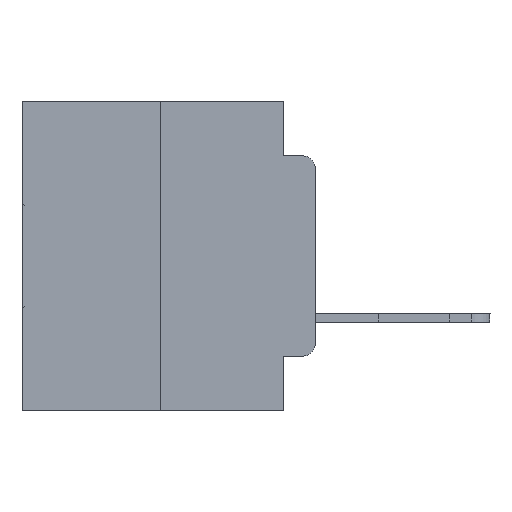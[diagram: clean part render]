
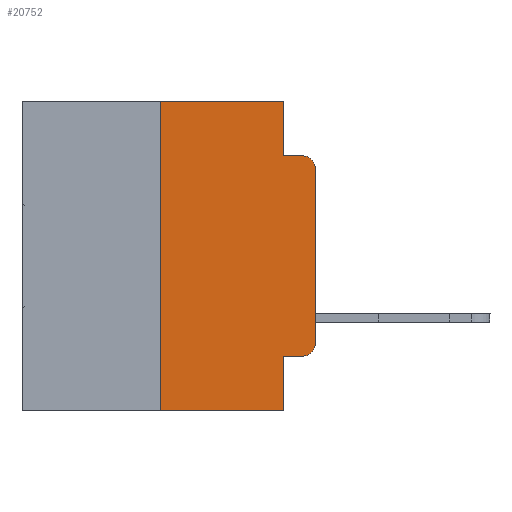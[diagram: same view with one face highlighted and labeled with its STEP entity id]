
A CAD part, left-side view. The second image highlights one B-rep face of the part: STEP entity #20752.
In plain terms, the highlighted planar face has unit normal (-1, 0, 0).
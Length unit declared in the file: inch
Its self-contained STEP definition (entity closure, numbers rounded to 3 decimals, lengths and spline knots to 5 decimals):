
#419 = CARTESIAN_POINT ( 'NONE',  ( 0., 0.25, 0. ) ) ;
#606 = CARTESIAN_POINT ( 'NONE',  ( 0., 0., -0.3915 ) ) ;
#669 = CARTESIAN_POINT ( 'NONE',  ( 0., 0.051, 0. ) ) ;
#804 = LINE ( 'NONE', #19775, #17486 ) ;
#951 = DIRECTION ( 'NONE',  ( 0., 0., 1. ) ) ;
#1592 = CIRCLE ( 'NONE', #18840, 0.02 ) ;
#1595 = VERTEX_POINT ( 'NONE', #11694 ) ;
#1695 = AXIS2_PLACEMENT_3D ( 'NONE', #17383, #21545, #22154 ) ;
#1738 = DIRECTION ( 'NONE',  ( 0., -1., 0. ) ) ;
#2549 = VERTEX_POINT ( 'NONE', #7487 ) ;
#3279 = DIRECTION ( 'NONE',  ( 0., -1., 0. ) ) ;
#3861 = LINE ( 'NONE', #10783, #11491 ) ;
#3958 = DIRECTION ( 'NONE',  ( 0., 0., -1. ) ) ;
#3966 = AXIS2_PLACEMENT_3D ( 'NONE', #23232, #30220, #18471 ) ;
#4271 = EDGE_CURVE ( 'NONE', #17627, #30252, #14531, .T. ) ;
#4440 = VECTOR ( 'NONE', #3279, 39.37008 ) ;
#4605 = EDGE_LOOP ( 'NONE', ( #21829, #26797, #7117, #13306, #5757, #14595, #7128, #30144, #10093, #21028 ) ) ;
#4985 = EDGE_CURVE ( 'NONE', #2549, #11562, #25563, .T. ) ;
#5744 = LINE ( 'NONE', #22222, #4440 ) ;
#5757 = ORIENTED_EDGE ( 'NONE', *, *, #18303, .F. ) ;
#5864 = VECTOR ( 'NONE', #15097, 39.37008 ) ;
#5902 = EDGE_CURVE ( 'NONE', #30252, #1595, #30450, .T. ) ;
#6828 = DIRECTION ( 'NONE',  ( 0., -1., 0. ) ) ;
#7117 = ORIENTED_EDGE ( 'NONE', *, *, #5902, .F. ) ;
#7128 = ORIENTED_EDGE ( 'NONE', *, *, #15483, .T. ) ;
#7487 = CARTESIAN_POINT ( 'NONE',  ( 0., 0.02, -0.4115 ) ) ;
#7666 = FACE_OUTER_BOUND ( 'NONE', #4605, .T. ) ;
#8427 = CARTESIAN_POINT ( 'NONE',  ( 0., 0.02, -0.1085 ) ) ;
#9106 = EDGE_CURVE ( 'NONE', #24714, #1595, #1592, .T. ) ;
#10093 = ORIENTED_EDGE ( 'NONE', *, *, #13105, .T. ) ;
#10783 = CARTESIAN_POINT ( 'NONE',  ( 0., 0.25, 0. ) ) ;
#10971 = CARTESIAN_POINT ( 'NONE',  ( 0., 0.473, -0.5 ) ) ;
#11491 = VECTOR ( 'NONE', #22671, 39.37008 ) ;
#11562 = VERTEX_POINT ( 'NONE', #606 ) ;
#11694 = CARTESIAN_POINT ( 'NONE',  ( 0., 0.02, -0.0885 ) ) ;
#11901 = DIRECTION ( 'NONE',  ( 0., 0., -1. ) ) ;
#13105 = EDGE_CURVE ( 'NONE', #18652, #2549, #23702, .T. ) ;
#13125 = LINE ( 'NONE', #10971, #24481 ) ;
#13184 = DIRECTION ( 'NONE',  ( -1., 0., 0. ) ) ;
#13306 = ORIENTED_EDGE ( 'NONE', *, *, #4271, .F. ) ;
#14531 = LINE ( 'NONE', #669, #15434 ) ;
#14595 = ORIENTED_EDGE ( 'NONE', *, *, #29845, .F. ) ;
#14738 = VERTEX_POINT ( 'NONE', #23242 ) ;
#15097 = DIRECTION ( 'NONE',  ( 0., 0., -1. ) ) ;
#15434 = VECTOR ( 'NONE', #11901, 39.37008 ) ;
#15483 = EDGE_CURVE ( 'NONE', #14738, #23573, #13125, .T. ) ;
#17383 = CARTESIAN_POINT ( 'NONE',  ( 0., 0.473, 0. ) ) ;
#17486 = VECTOR ( 'NONE', #951, 39.37008 ) ;
#17608 = EDGE_CURVE ( 'NONE', #18652, #23573, #29475, .T. ) ;
#17627 = VERTEX_POINT ( 'NONE', #18025 ) ;
#18025 = CARTESIAN_POINT ( 'NONE',  ( 0., 0.051, 0. ) ) ;
#18303 = EDGE_CURVE ( 'NONE', #20727, #17627, #5744, .T. ) ;
#18471 = DIRECTION ( 'NONE',  ( 0., 0., -1. ) ) ;
#18652 = VERTEX_POINT ( 'NONE', #22065 ) ;
#18840 = AXIS2_PLACEMENT_3D ( 'NONE', #8427, #13184, #3958 ) ;
#18935 = CARTESIAN_POINT ( 'NONE',  ( 0., 0.051, -0.4115 ) ) ;
#19544 = VECTOR ( 'NONE', #28371, 39.37008 ) ;
#19775 = CARTESIAN_POINT ( 'NONE',  ( 0., 0., 0. ) ) ;
#20727 = VERTEX_POINT ( 'NONE', #419 ) ;
#20752 = ADVANCED_FACE ( 'NONE', ( #7666 ), #28982, .F. ) ;
#21028 = ORIENTED_EDGE ( 'NONE', *, *, #4985, .T. ) ;
#21190 = EDGE_CURVE ( 'NONE', #11562, #24714, #804, .T. ) ;
#21545 = DIRECTION ( 'NONE',  ( 1., 0., 0. ) ) ;
#21829 = ORIENTED_EDGE ( 'NONE', *, *, #21190, .T. ) ;
#22065 = CARTESIAN_POINT ( 'NONE',  ( 0., 0.051, -0.4115 ) ) ;
#22154 = DIRECTION ( 'NONE',  ( 0., 0., -1. ) ) ;
#22222 = CARTESIAN_POINT ( 'NONE',  ( 0., 0.473, 0. ) ) ;
#22648 = CARTESIAN_POINT ( 'NONE',  ( 0., 0.051, 0. ) ) ;
#22671 = DIRECTION ( 'NONE',  ( 0., 0., 1. ) ) ;
#23159 = CARTESIAN_POINT ( 'NONE',  ( 0., 0.051, -0.0885 ) ) ;
#23232 = CARTESIAN_POINT ( 'NONE',  ( 0., 0.02, -0.3915 ) ) ;
#23242 = CARTESIAN_POINT ( 'NONE',  ( 0., 0.25, -0.5 ) ) ;
#23573 = VERTEX_POINT ( 'NONE', #25425 ) ;
#23702 = LINE ( 'NONE', #18935, #19544 ) ;
#24481 = VECTOR ( 'NONE', #1738, 39.37008 ) ;
#24714 = VERTEX_POINT ( 'NONE', #30085 ) ;
#25274 = CARTESIAN_POINT ( 'NONE',  ( 0., 0.051, -0.0885 ) ) ;
#25425 = CARTESIAN_POINT ( 'NONE',  ( 0., 0.051, -0.5 ) ) ;
#25563 = CIRCLE ( 'NONE', #3966, 0.02 ) ;
#26797 = ORIENTED_EDGE ( 'NONE', *, *, #9106, .T. ) ;
#27927 = VECTOR ( 'NONE', #6828, 39.37008 ) ;
#28371 = DIRECTION ( 'NONE',  ( 0., -1., 0. ) ) ;
#28982 = PLANE ( 'NONE',  #1695 ) ;
#29475 = LINE ( 'NONE', #22648, #5864 ) ;
#29845 = EDGE_CURVE ( 'NONE', #14738, #20727, #3861, .T. ) ;
#30085 = CARTESIAN_POINT ( 'NONE',  ( 0., 0., -0.1085 ) ) ;
#30144 = ORIENTED_EDGE ( 'NONE', *, *, #17608, .F. ) ;
#30220 = DIRECTION ( 'NONE',  ( -1., 0., 0. ) ) ;
#30252 = VERTEX_POINT ( 'NONE', #25274 ) ;
#30450 = LINE ( 'NONE', #23159, #27927 ) ;
